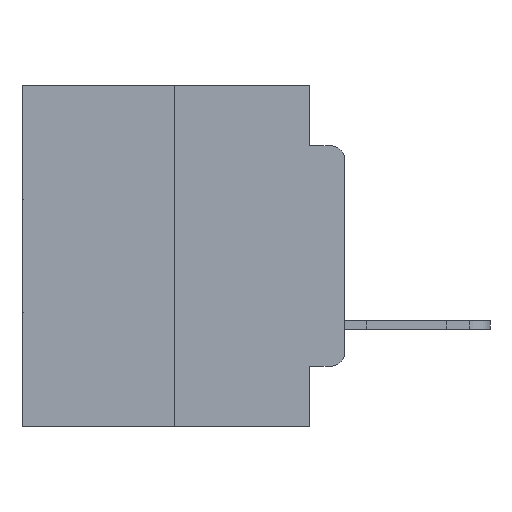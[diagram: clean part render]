
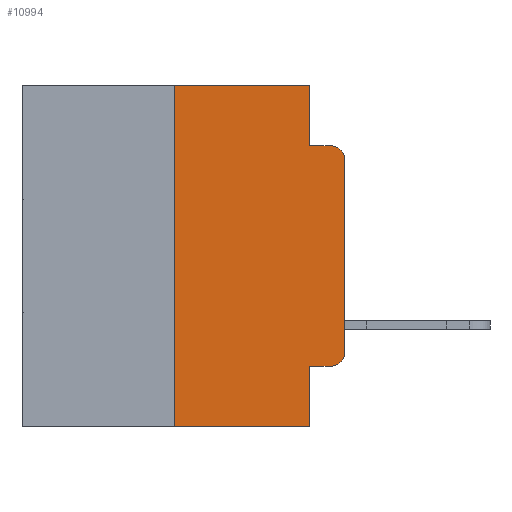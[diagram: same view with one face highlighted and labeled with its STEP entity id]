
A CAD part, left-side view. The second image highlights one B-rep face of the part: STEP entity #10994.
In plain terms, the highlighted planar face has unit normal (-1, 0, 0).
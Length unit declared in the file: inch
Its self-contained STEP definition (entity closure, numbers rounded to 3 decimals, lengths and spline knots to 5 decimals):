
#39 = CARTESIAN_POINT ( 'NONE',  ( 0., 0.051, 0. ) ) ;
#457 = VERTEX_POINT ( 'NONE', #15091 ) ;
#460 = ORIENTED_EDGE ( 'NONE', *, *, #15081, .F. ) ;
#639 = DIRECTION ( 'NONE',  ( 0., 0., -1. ) ) ;
#1960 = FACE_OUTER_BOUND ( 'NONE', #11149, .T. ) ;
#2013 = CARTESIAN_POINT ( 'NONE',  ( 0., 0., 0. ) ) ;
#3171 = CARTESIAN_POINT ( 'NONE',  ( 0., 0.25, 0. ) ) ;
#3195 = ORIENTED_EDGE ( 'NONE', *, *, #6811, .T. ) ;
#3504 = VERTEX_POINT ( 'NONE', #13472 ) ;
#3605 = VECTOR ( 'NONE', #639, 39.37008 ) ;
#3936 = VECTOR ( 'NONE', #23544, 39.37008 ) ;
#4088 = DIRECTION ( 'NONE',  ( 0., -1., 0. ) ) ;
#4354 = CIRCLE ( 'NONE', #13947, 0.02 ) ;
#5068 = CARTESIAN_POINT ( 'NONE',  ( 0., 0.25, -0.5 ) ) ;
#5745 = DIRECTION ( 'NONE',  ( 0., 0., -1. ) ) ;
#5754 = DIRECTION ( 'NONE',  ( -1., 0., 0. ) ) ;
#5816 = CARTESIAN_POINT ( 'NONE',  ( 0., 0.02, -0.1085 ) ) ;
#6295 = VECTOR ( 'NONE', #23929, 39.37008 ) ;
#6811 = EDGE_CURVE ( 'NONE', #24010, #3504, #10727, .T. ) ;
#7380 = LINE ( 'NONE', #14701, #22009 ) ;
#7544 = VERTEX_POINT ( 'NONE', #19558 ) ;
#7980 = EDGE_CURVE ( 'NONE', #7544, #13122, #27041, .T. ) ;
#8189 = CARTESIAN_POINT ( 'NONE',  ( 0., 0.051, 0. ) ) ;
#8757 = DIRECTION ( 'NONE',  ( 0., 0., 1. ) ) ;
#9025 = DIRECTION ( 'NONE',  ( 0., 0., 1. ) ) ;
#9112 = CARTESIAN_POINT ( 'NONE',  ( 0., 0.25, 0. ) ) ;
#9826 = CARTESIAN_POINT ( 'NONE',  ( 0., 0.02, -0.0885 ) ) ;
#9839 = VERTEX_POINT ( 'NONE', #3171 ) ;
#10217 = LINE ( 'NONE', #23740, #3936 ) ;
#10268 = ORIENTED_EDGE ( 'NONE', *, *, #14104, .F. ) ;
#10635 = LINE ( 'NONE', #39, #3605 ) ;
#10727 = LINE ( 'NONE', #2013, #11452 ) ;
#10767 = EDGE_CURVE ( 'NONE', #17241, #21343, #10217, .T. ) ;
#10994 = ADVANCED_FACE ( 'NONE', ( #1960 ), #20496, .F. ) ;
#11149 = EDGE_LOOP ( 'NONE', ( #3195, #15404, #10268, #21089, #21700, #17191, #27045, #460, #24120, #24687 ) ) ;
#11452 = VECTOR ( 'NONE', #8757, 39.37008 ) ;
#11704 = VECTOR ( 'NONE', #4088, 39.37008 ) ;
#11982 = EDGE_CURVE ( 'NONE', #3504, #12524, #15296, .T. ) ;
#12524 = VERTEX_POINT ( 'NONE', #9826 ) ;
#13122 = VERTEX_POINT ( 'NONE', #15069 ) ;
#13472 = CARTESIAN_POINT ( 'NONE',  ( 0., 0., -0.1085 ) ) ;
#13947 = AXIS2_PLACEMENT_3D ( 'NONE', #26126, #26081, #26053 ) ;
#14104 = EDGE_CURVE ( 'NONE', #457, #12524, #17874, .T. ) ;
#14162 = EDGE_CURVE ( 'NONE', #9839, #17011, #21149, .T. ) ;
#14448 = DIRECTION ( 'NONE',  ( 0., 0., -1. ) ) ;
#14535 = EDGE_CURVE ( 'NONE', #17011, #457, #7380, .T. ) ;
#14701 = CARTESIAN_POINT ( 'NONE',  ( 0., 0.051, 0. ) ) ;
#14739 = EDGE_CURVE ( 'NONE', #17241, #9839, #27060, .T. ) ;
#15069 = CARTESIAN_POINT ( 'NONE',  ( 0., 0.02, -0.4115 ) ) ;
#15081 = EDGE_CURVE ( 'NONE', #7544, #21343, #10635, .T. ) ;
#15091 = CARTESIAN_POINT ( 'NONE',  ( 0., 0.051, -0.0885 ) ) ;
#15095 = EDGE_CURVE ( 'NONE', #13122, #24010, #4354, .T. ) ;
#15144 = CARTESIAN_POINT ( 'NONE',  ( 0., 0.051, -0.4115 ) ) ;
#15296 = CIRCLE ( 'NONE', #26415, 0.02 ) ;
#15404 = ORIENTED_EDGE ( 'NONE', *, *, #11982, .T. ) ;
#15882 = CARTESIAN_POINT ( 'NONE',  ( 0., 0.051, -0.5 ) ) ;
#17011 = VERTEX_POINT ( 'NONE', #8189 ) ;
#17191 = ORIENTED_EDGE ( 'NONE', *, *, #14739, .F. ) ;
#17241 = VERTEX_POINT ( 'NONE', #5068 ) ;
#17344 = AXIS2_PLACEMENT_3D ( 'NONE', #20531, #20427, #20423 ) ;
#17874 = LINE ( 'NONE', #24855, #6295 ) ;
#19558 = CARTESIAN_POINT ( 'NONE',  ( 0., 0.051, -0.4115 ) ) ;
#20423 = DIRECTION ( 'NONE',  ( 0., 0., -1. ) ) ;
#20427 = DIRECTION ( 'NONE',  ( 1., 0., 0. ) ) ;
#20496 = PLANE ( 'NONE',  #17344 ) ;
#20531 = CARTESIAN_POINT ( 'NONE',  ( 0., 0.473, 0. ) ) ;
#20962 = CARTESIAN_POINT ( 'NONE',  ( 0., 0., -0.3915 ) ) ;
#21089 = ORIENTED_EDGE ( 'NONE', *, *, #14535, .F. ) ;
#21149 = LINE ( 'NONE', #22623, #25527 ) ;
#21343 = VERTEX_POINT ( 'NONE', #15882 ) ;
#21700 = ORIENTED_EDGE ( 'NONE', *, *, #14162, .F. ) ;
#22009 = VECTOR ( 'NONE', #14448, 39.37008 ) ;
#22310 = VECTOR ( 'NONE', #9025, 39.37008 ) ;
#22623 = CARTESIAN_POINT ( 'NONE',  ( 0., 0.473, 0. ) ) ;
#22704 = DIRECTION ( 'NONE',  ( 0., -1., 0. ) ) ;
#23544 = DIRECTION ( 'NONE',  ( 0., -1., 0. ) ) ;
#23740 = CARTESIAN_POINT ( 'NONE',  ( 0., 0.473, -0.5 ) ) ;
#23929 = DIRECTION ( 'NONE',  ( 0., -1., 0. ) ) ;
#24010 = VERTEX_POINT ( 'NONE', #20962 ) ;
#24120 = ORIENTED_EDGE ( 'NONE', *, *, #7980, .T. ) ;
#24687 = ORIENTED_EDGE ( 'NONE', *, *, #15095, .T. ) ;
#24855 = CARTESIAN_POINT ( 'NONE',  ( 0., 0.051, -0.0885 ) ) ;
#25527 = VECTOR ( 'NONE', #22704, 39.37008 ) ;
#26053 = DIRECTION ( 'NONE',  ( 0., 0., -1. ) ) ;
#26081 = DIRECTION ( 'NONE',  ( -1., 0., 0. ) ) ;
#26126 = CARTESIAN_POINT ( 'NONE',  ( 0., 0.02, -0.3915 ) ) ;
#26415 = AXIS2_PLACEMENT_3D ( 'NONE', #5816, #5754, #5745 ) ;
#27041 = LINE ( 'NONE', #15144, #11704 ) ;
#27045 = ORIENTED_EDGE ( 'NONE', *, *, #10767, .T. ) ;
#27060 = LINE ( 'NONE', #9112, #22310 ) ;
